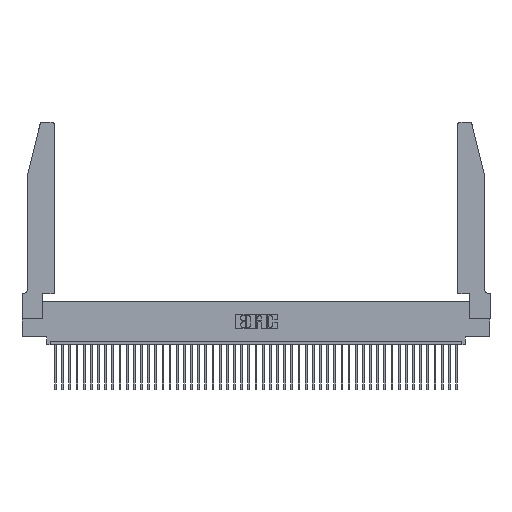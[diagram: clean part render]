
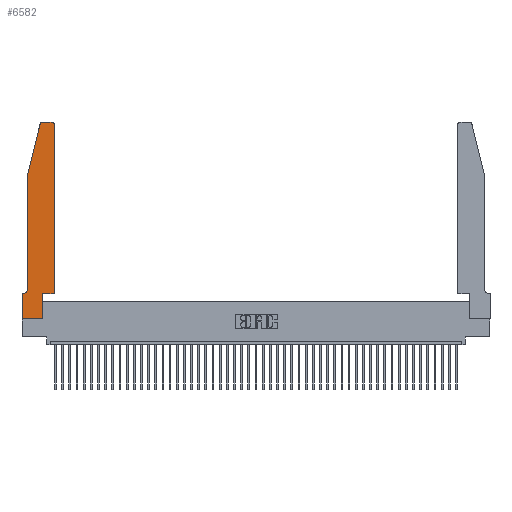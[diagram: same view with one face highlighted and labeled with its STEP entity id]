
A CAD part, top view. The second image highlights one B-rep face of the part: STEP entity #6582.
In plain terms, the highlighted planar face has unit normal (0, 0, 1).
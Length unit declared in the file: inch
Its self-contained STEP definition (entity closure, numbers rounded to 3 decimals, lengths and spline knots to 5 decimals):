
#458 = VERTEX_POINT ( 'NONE', #22380 ) ;
#1550 = VERTEX_POINT ( 'NONE', #31583 ) ;
#1616 = CARTESIAN_POINT ( 'NONE',  ( 0.0055, 0.42, 0.37 ) ) ;
#1818 = VECTOR ( 'NONE', #43378, 39.37008 ) ;
#1867 = VERTEX_POINT ( 'NONE', #44210 ) ;
#1871 = CARTESIAN_POINT ( 'NONE',  ( 0., 0., 0.37 ) ) ;
#2012 = EDGE_LOOP ( 'NONE', ( #31071, #43120, #39912, #35375, #33541, #44999, #12804, #3893, #36593, #4622, #8595, #7467 ) ) ;
#2903 = DIRECTION ( 'NONE',  ( 1., 0., 0. ) ) ;
#3048 = VERTEX_POINT ( 'NONE', #1871 ) ;
#3495 = DIRECTION ( 'NONE',  ( 0., 1., 0. ) ) ;
#3893 = ORIENTED_EDGE ( 'NONE', *, *, #43065, .T. ) ;
#4622 = ORIENTED_EDGE ( 'NONE', *, *, #33158, .T. ) ;
#4709 = DIRECTION ( 'NONE',  ( 0., 0., -1. ) ) ;
#4825 = VERTEX_POINT ( 'NONE', #13795 ) ;
#4913 = LINE ( 'NONE', #16450, #8204 ) ;
#5465 = EDGE_CURVE ( 'NONE', #1867, #458, #32744, .T. ) ;
#5857 = DIRECTION ( 'NONE',  ( 0., 0., 1. ) ) ;
#6572 = DIRECTION ( 'NONE',  ( 0., 0., 1. ) ) ;
#6582 = ADVANCED_FACE ( 'NONE', ( #43168 ), #45468, .T. ) ;
#6937 = EDGE_CURVE ( 'NONE', #9380, #16133, #32051, .T. ) ;
#7467 = ORIENTED_EDGE ( 'NONE', *, *, #5465, .T. ) ;
#8204 = VECTOR ( 'NONE', #9355, 39.37008 ) ;
#8595 = ORIENTED_EDGE ( 'NONE', *, *, #9204, .T. ) ;
#8961 = EDGE_CURVE ( 'NONE', #1550, #3048, #29493, .T. ) ;
#9204 = EDGE_CURVE ( 'NONE', #36550, #1867, #30628, .T. ) ;
#9355 = DIRECTION ( 'NONE',  ( -1., 0., 0. ) ) ;
#9380 = VERTEX_POINT ( 'NONE', #37742 ) ;
#9778 = DIRECTION ( 'NONE',  ( 0., -1., 0. ) ) ;
#10083 = CARTESIAN_POINT ( 'NONE',  ( 0.0755, 2., 0.37 ) ) ;
#10391 = LINE ( 'NONE', #14847, #18064 ) ;
#10631 = CARTESIAN_POINT ( 'NONE',  ( 0.2865, 0.35, 0.37 ) ) ;
#12073 = DIRECTION ( 'NONE',  ( -1., 0., 0. ) ) ;
#12200 = DIRECTION ( 'NONE',  ( 0., -1., 0. ) ) ;
#12804 = ORIENTED_EDGE ( 'NONE', *, *, #8961, .T. ) ;
#12825 = LINE ( 'NONE', #24484, #35527 ) ;
#13281 = VECTOR ( 'NONE', #17008, 39.37008 ) ;
#13342 = CARTESIAN_POINT ( 'NONE',  ( 0.4205, 2.72, 0.37 ) ) ;
#13780 = CARTESIAN_POINT ( 'NONE',  ( 0., 0., 0.37 ) ) ;
#13795 = CARTESIAN_POINT ( 'NONE',  ( 0.2865, 0., 0.37 ) ) ;
#14232 = CARTESIAN_POINT ( 'NONE',  ( 0.0055, 0.35, 0.37 ) ) ;
#14355 = AXIS2_PLACEMENT_3D ( 'NONE', #24607, #20424, #24318 ) ;
#14847 = CARTESIAN_POINT ( 'NONE',  ( 0., 0., 0.37 ) ) ;
#14878 = DIRECTION ( 'NONE',  ( 1., 0., 0. ) ) ;
#16133 = VERTEX_POINT ( 'NONE', #19731 ) ;
#16450 = CARTESIAN_POINT ( 'NONE',  ( 0.2605, 2.75, 0.37 ) ) ;
#17008 = DIRECTION ( 'NONE',  ( -0.239, -0.971, 0. ) ) ;
#17283 = AXIS2_PLACEMENT_3D ( 'NONE', #13342, #5857, #14878 ) ;
#18064 = VECTOR ( 'NONE', #18546, 39.37008 ) ;
#18520 = VERTEX_POINT ( 'NONE', #45776 ) ;
#18546 = DIRECTION ( 'NONE',  ( 1., 0., 0. ) ) ;
#19731 = CARTESIAN_POINT ( 'NONE',  ( 0.0755, 2., 0.37 ) ) ;
#20424 = DIRECTION ( 'NONE',  ( 0., 0., 1. ) ) ;
#20635 = VERTEX_POINT ( 'NONE', #27391 ) ;
#20801 = CIRCLE ( 'NONE', #38419, 0.07 ) ;
#21108 = VERTEX_POINT ( 'NONE', #10631 ) ;
#21177 = VECTOR ( 'NONE', #25250, 39.37008 ) ;
#22249 = LINE ( 'NONE', #29243, #44415 ) ;
#22380 = CARTESIAN_POINT ( 'NONE',  ( 0.4205, 2.75, 0.37 ) ) ;
#22519 = CARTESIAN_POINT ( 'NONE',  ( 0.4505, 0.35, 0.37 ) ) ;
#22562 = EDGE_CURVE ( 'NONE', #16133, #20635, #22249, .T. ) ;
#22864 = EDGE_CURVE ( 'NONE', #28249, #1550, #34978, .T. ) ;
#23426 = VECTOR ( 'NONE', #9778, 39.37008 ) ;
#24318 = DIRECTION ( 'NONE',  ( 1., 0., 0. ) ) ;
#24484 = CARTESIAN_POINT ( 'NONE',  ( 0.2865, 0.35, 0.37 ) ) ;
#24607 = CARTESIAN_POINT ( 'NONE',  ( 0., 0.35, 0.37 ) ) ;
#25250 = DIRECTION ( 'NONE',  ( 0., 1., 0. ) ) ;
#25432 = CARTESIAN_POINT ( 'NONE',  ( 0.4505, 0.35, 0.37 ) ) ;
#27391 = CARTESIAN_POINT ( 'NONE',  ( 0.0755, 0.42, 0.37 ) ) ;
#28249 = VERTEX_POINT ( 'NONE', #14232 ) ;
#28348 = CARTESIAN_POINT ( 'NONE',  ( 0.4505, 0.35, 0.37 ) ) ;
#29090 = AXIS2_PLACEMENT_3D ( 'NONE', #35162, #6572, #2903 ) ;
#29243 = CARTESIAN_POINT ( 'NONE',  ( 0.0755, 2., 0.37 ) ) ;
#29493 = LINE ( 'NONE', #13780, #23426 ) ;
#29716 = EDGE_CURVE ( 'NONE', #20635, #28249, #20801, .T. ) ;
#30628 = LINE ( 'NONE', #28348, #21177 ) ;
#31034 = LINE ( 'NONE', #25432, #42600 ) ;
#31071 = ORIENTED_EDGE ( 'NONE', *, *, #42597, .T. ) ;
#31583 = CARTESIAN_POINT ( 'NONE',  ( 0., 0.35, 0.37 ) ) ;
#32051 = LINE ( 'NONE', #10083, #13281 ) ;
#32744 = CIRCLE ( 'NONE', #17283, 0.03 ) ;
#33158 = EDGE_CURVE ( 'NONE', #21108, #36550, #31034, .T. ) ;
#33541 = ORIENTED_EDGE ( 'NONE', *, *, #29716, .T. ) ;
#34978 = LINE ( 'NONE', #43712, #1818 ) ;
#35162 = CARTESIAN_POINT ( 'NONE',  ( 0.284, 2.72, 0.37 ) ) ;
#35375 = ORIENTED_EDGE ( 'NONE', *, *, #22562, .T. ) ;
#35527 = VECTOR ( 'NONE', #3495, 39.37008 ) ;
#36076 = DIRECTION ( 'NONE',  ( 1., 0., 0. ) ) ;
#36550 = VERTEX_POINT ( 'NONE', #22519 ) ;
#36593 = ORIENTED_EDGE ( 'NONE', *, *, #40630, .T. ) ;
#37742 = CARTESIAN_POINT ( 'NONE',  ( 0.25487, 2.72718, 0.37 ) ) ;
#38419 = AXIS2_PLACEMENT_3D ( 'NONE', #1616, #4709, #12073 ) ;
#39912 = ORIENTED_EDGE ( 'NONE', *, *, #6937, .T. ) ;
#40630 = EDGE_CURVE ( 'NONE', #4825, #21108, #12825, .T. ) ;
#42597 = EDGE_CURVE ( 'NONE', #458, #18520, #4913, .T. ) ;
#42600 = VECTOR ( 'NONE', #36076, 39.37008 ) ;
#42703 = EDGE_CURVE ( 'NONE', #18520, #9380, #45799, .T. ) ;
#43065 = EDGE_CURVE ( 'NONE', #3048, #4825, #10391, .T. ) ;
#43120 = ORIENTED_EDGE ( 'NONE', *, *, #42703, .T. ) ;
#43168 = FACE_OUTER_BOUND ( 'NONE', #2012, .T. ) ;
#43378 = DIRECTION ( 'NONE',  ( -1., 0., 0. ) ) ;
#43712 = CARTESIAN_POINT ( 'NONE',  ( 0.0755, 0.35, 0.37 ) ) ;
#44210 = CARTESIAN_POINT ( 'NONE',  ( 0.4505, 2.72, 0.37 ) ) ;
#44415 = VECTOR ( 'NONE', #12200, 39.37008 ) ;
#44999 = ORIENTED_EDGE ( 'NONE', *, *, #22864, .T. ) ;
#45468 = PLANE ( 'NONE',  #14355 ) ;
#45776 = CARTESIAN_POINT ( 'NONE',  ( 0.284, 2.75, 0.37 ) ) ;
#45799 = CIRCLE ( 'NONE', #29090, 0.03 ) ;
